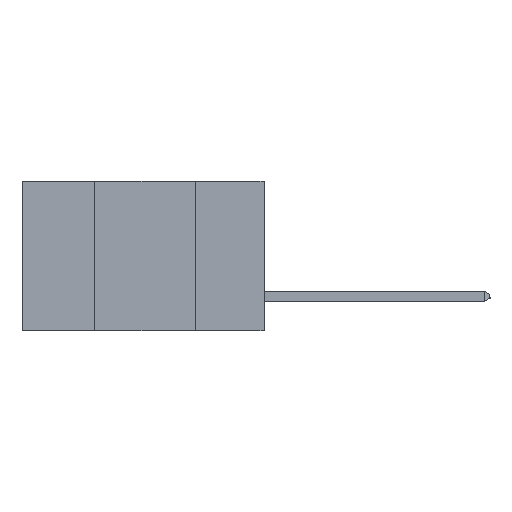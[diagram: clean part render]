
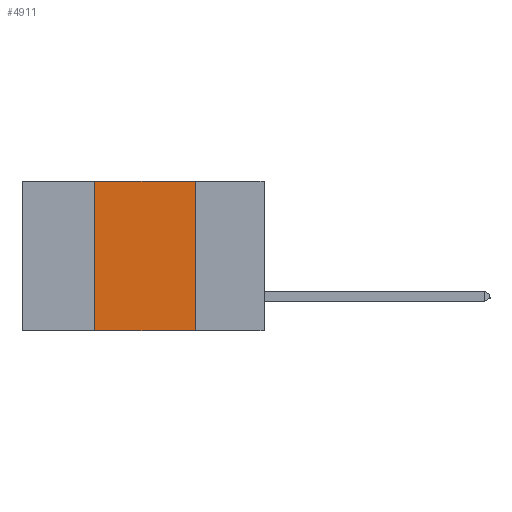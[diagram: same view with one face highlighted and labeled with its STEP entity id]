
A CAD part, left-side view. The second image highlights one B-rep face of the part: STEP entity #4911.
In plain terms, the highlighted planar face has unit normal (-1, 0, 0).
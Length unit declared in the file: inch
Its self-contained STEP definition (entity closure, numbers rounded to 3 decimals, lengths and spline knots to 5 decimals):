
#131 = ORIENTED_EDGE ( 'NONE', *, *, #12241, .F. ) ;
#648 = VECTOR ( 'NONE', #11751, 39.37008 ) ;
#933 = CARTESIAN_POINT ( 'NONE',  ( 0., 0.6, 0. ) ) ;
#965 = DIRECTION ( 'NONE',  ( 0., 0., -1. ) ) ;
#980 = CARTESIAN_POINT ( 'NONE',  ( 0., 0.42, -0.37 ) ) ;
#1531 = CARTESIAN_POINT ( 'NONE',  ( 0., 0.17, -0.37 ) ) ;
#1642 = VERTEX_POINT ( 'NONE', #9727 ) ;
#2283 = VECTOR ( 'NONE', #8202, 39.37008 ) ;
#2578 = VECTOR ( 'NONE', #11409, 39.37008 ) ;
#2800 = CARTESIAN_POINT ( 'NONE',  ( 0., 0.6, 0. ) ) ;
#3794 = DIRECTION ( 'NONE',  ( 0., 0., -1. ) ) ;
#3889 = CARTESIAN_POINT ( 'NONE',  ( 0., 0.17, 0. ) ) ;
#4326 = VERTEX_POINT ( 'NONE', #980 ) ;
#4342 = AXIS2_PLACEMENT_3D ( 'NONE', #2800, #9503, #3794 ) ;
#4624 = EDGE_CURVE ( 'NONE', #4326, #1642, #10202, .T. ) ;
#4911 = ADVANCED_FACE ( 'NONE', ( #11867 ), #7623, .F. ) ;
#5185 = LINE ( 'NONE', #933, #2578 ) ;
#5259 = CARTESIAN_POINT ( 'NONE',  ( 0., 0.6, -0.37 ) ) ;
#6481 = VERTEX_POINT ( 'NONE', #3889 ) ;
#6708 = ORIENTED_EDGE ( 'NONE', *, *, #10305, .F. ) ;
#7623 = PLANE ( 'NONE',  #4342 ) ;
#8170 = VERTEX_POINT ( 'NONE', #1531 ) ;
#8202 = DIRECTION ( 'NONE',  ( 0., 0., 1. ) ) ;
#8654 = ORIENTED_EDGE ( 'NONE', *, *, #8709, .T. ) ;
#8709 = EDGE_CURVE ( 'NONE', #4326, #8170, #10821, .T. ) ;
#9230 = LINE ( 'NONE', #12313, #11323 ) ;
#9503 = DIRECTION ( 'NONE',  ( 1., 0., 0. ) ) ;
#9727 = CARTESIAN_POINT ( 'NONE',  ( 0., 0.42, 0. ) ) ;
#10050 = CARTESIAN_POINT ( 'NONE',  ( 0., 0.42, 0. ) ) ;
#10202 = LINE ( 'NONE', #10050, #2283 ) ;
#10305 = EDGE_CURVE ( 'NONE', #6481, #8170, #9230, .T. ) ;
#10821 = LINE ( 'NONE', #5259, #648 ) ;
#10903 = EDGE_LOOP ( 'NONE', ( #6708, #131, #12171, #8654 ) ) ;
#11323 = VECTOR ( 'NONE', #965, 39.37008 ) ;
#11409 = DIRECTION ( 'NONE',  ( 0., -1., 0. ) ) ;
#11751 = DIRECTION ( 'NONE',  ( 0., -1., 0. ) ) ;
#11867 = FACE_OUTER_BOUND ( 'NONE', #10903, .T. ) ;
#12171 = ORIENTED_EDGE ( 'NONE', *, *, #4624, .F. ) ;
#12241 = EDGE_CURVE ( 'NONE', #1642, #6481, #5185, .T. ) ;
#12313 = CARTESIAN_POINT ( 'NONE',  ( 0., 0.17, 0. ) ) ;
